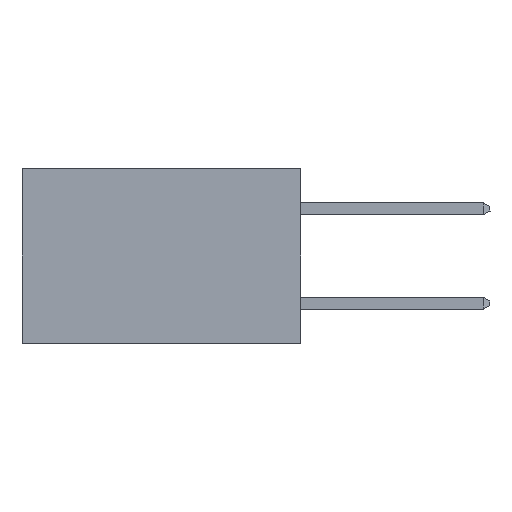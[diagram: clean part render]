
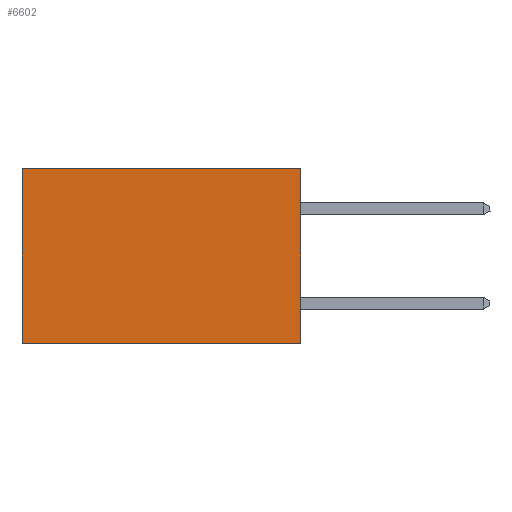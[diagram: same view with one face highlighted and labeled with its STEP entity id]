
A CAD part, left-side view. The second image highlights one B-rep face of the part: STEP entity #6602.
In plain terms, the highlighted planar face has unit normal (-1, 0, 0).
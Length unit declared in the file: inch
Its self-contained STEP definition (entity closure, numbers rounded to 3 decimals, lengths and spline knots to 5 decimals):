
#282 = VECTOR ( 'NONE', #7257, 39.37008 ) ;
#534 = ORIENTED_EDGE ( 'NONE', *, *, #15648, .F. ) ;
#852 = VECTOR ( 'NONE', #13886, 39.37008 ) ;
#1300 = ORIENTED_EDGE ( 'NONE', *, *, #3830, .T. ) ;
#2255 = LINE ( 'NONE', #15158, #16955 ) ;
#2956 = DIRECTION ( 'NONE',  ( 0., 0., -1. ) ) ;
#2973 = DIRECTION ( 'NONE',  ( 1., 0., 0. ) ) ;
#3830 = EDGE_CURVE ( 'NONE', #13550, #7017, #10046, .T. ) ;
#4318 = AXIS2_PLACEMENT_3D ( 'NONE', #11448, #2973, #2956 ) ;
#4606 = LINE ( 'NONE', #7623, #282 ) ;
#4705 = EDGE_CURVE ( 'NONE', #7017, #14392, #8632, .T. ) ;
#5230 = VECTOR ( 'NONE', #12618, 39.37008 ) ;
#6602 = ADVANCED_FACE ( 'NONE', ( #17982 ), #17204, .F. ) ;
#7017 = VERTEX_POINT ( 'NONE', #7605 ) ;
#7257 = DIRECTION ( 'NONE',  ( 0., 1., 0. ) ) ;
#7605 = CARTESIAN_POINT ( 'NONE',  ( 0.277, 0.59, 0. ) ) ;
#7623 = CARTESIAN_POINT ( 'NONE',  ( 0.277, 0., -0.37 ) ) ;
#7814 = DIRECTION ( 'NONE',  ( 0., 0., -1. ) ) ;
#8087 = VERTEX_POINT ( 'NONE', #9266 ) ;
#8632 = LINE ( 'NONE', #13044, #852 ) ;
#8987 = CARTESIAN_POINT ( 'NONE',  ( 0.277, 0., 0. ) ) ;
#9266 = CARTESIAN_POINT ( 'NONE',  ( 0.277, 0., -0.37 ) ) ;
#10046 = LINE ( 'NONE', #16274, #5230 ) ;
#10827 = EDGE_LOOP ( 'NONE', ( #12794, #13897, #534, #1300 ) ) ;
#11448 = CARTESIAN_POINT ( 'NONE',  ( 0.277, 0., -0.37 ) ) ;
#12087 = EDGE_CURVE ( 'NONE', #8087, #14392, #4606, .T. ) ;
#12618 = DIRECTION ( 'NONE',  ( 0., 1., 0. ) ) ;
#12794 = ORIENTED_EDGE ( 'NONE', *, *, #4705, .T. ) ;
#13044 = CARTESIAN_POINT ( 'NONE',  ( 0.277, 0.59, -0.37 ) ) ;
#13550 = VERTEX_POINT ( 'NONE', #8987 ) ;
#13886 = DIRECTION ( 'NONE',  ( 0., 0., -1. ) ) ;
#13897 = ORIENTED_EDGE ( 'NONE', *, *, #12087, .F. ) ;
#14392 = VERTEX_POINT ( 'NONE', #16625 ) ;
#15158 = CARTESIAN_POINT ( 'NONE',  ( 0.277, 0., -0.37 ) ) ;
#15648 = EDGE_CURVE ( 'NONE', #13550, #8087, #2255, .T. ) ;
#16274 = CARTESIAN_POINT ( 'NONE',  ( 0.277, 0., 0. ) ) ;
#16625 = CARTESIAN_POINT ( 'NONE',  ( 0.277, 0.59, -0.37 ) ) ;
#16955 = VECTOR ( 'NONE', #7814, 39.37008 ) ;
#17204 = PLANE ( 'NONE',  #4318 ) ;
#17982 = FACE_OUTER_BOUND ( 'NONE', #10827, .T. ) ;
